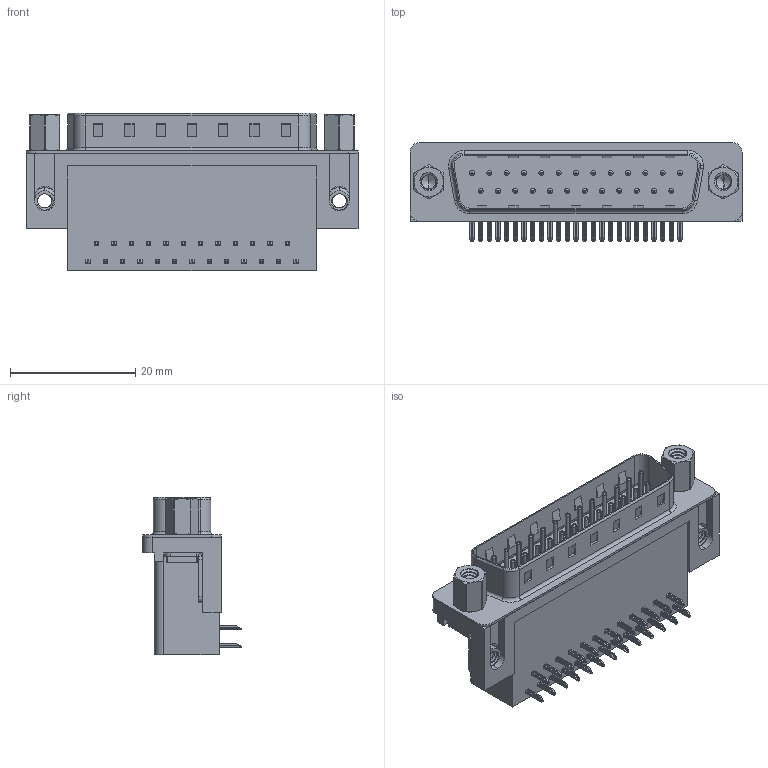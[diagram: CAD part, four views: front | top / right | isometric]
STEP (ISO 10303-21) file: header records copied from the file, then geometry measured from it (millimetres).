
FILE_DESCRIPTION (( 'STEP AP203' ), '1' );
FILE_NAME ('625-025-262-553.STEP', '2018-11-06T02:00:37', ( '' ), ( '' ), 'SwSTEP 2.0', 'SolidWorks 2016', '' );
FILE_SCHEMA (( 'CONFIG_CONTROL_DESIGN' ));
Length unit declared in the file: millimetre
Products named in the file (8): 625 Contact Bottom; 625 Contact Top; 625 4-40 Threaded Board Mount; 625 4-40 Threaded Rivet; 625 4-40 Hex Standoff 5; 625-025-262-553; 625 Housing_25 Socket; 625 Shell_25 Socket
Assembly tree (33 placements, depth 2):
  625-025-262-553
    625 Housing_25 Socket
    625 Shell_25 Socket
    625 Contact Bottom  x12
    625 Contact Top  x13
    625 4-40 Threaded Board Mount  x2
    625 4-40 Threaded Rivet  x2
    625 4-40 Hex Standoff 5  x2
Bounding box: 53.04 x 15.73 x 25.16 mm (x, y, z)
Volume: 9388.7 mm3; surface area: 9423.9 mm2
Topology: 33 solids, 33 shells, 2423 faces, 6047 edges, 3749 vertices
Faces by surface type: plane 1429, cylinder 745, torus 193, cone 32, bspline 24
Entity records: 29334 total; most frequent: CARTESIAN_POINT 9955, ORIENTED_EDGE 3708, DIRECTION 3694, EDGE_CURVE 1854, AXIS2_PLACEMENT_3D 1241, VECTOR 1212, LINE 1212, VERTEX_POINT 1192
